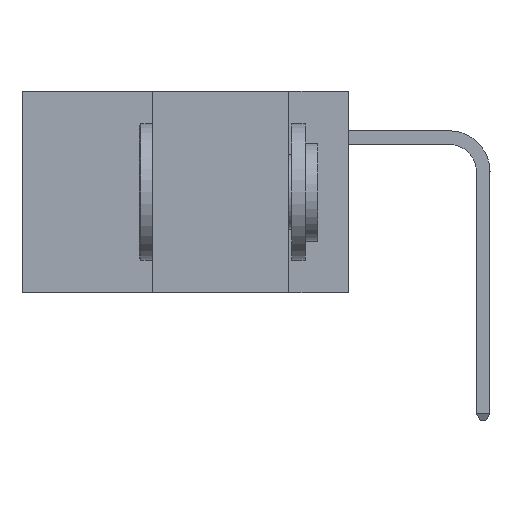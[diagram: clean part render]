
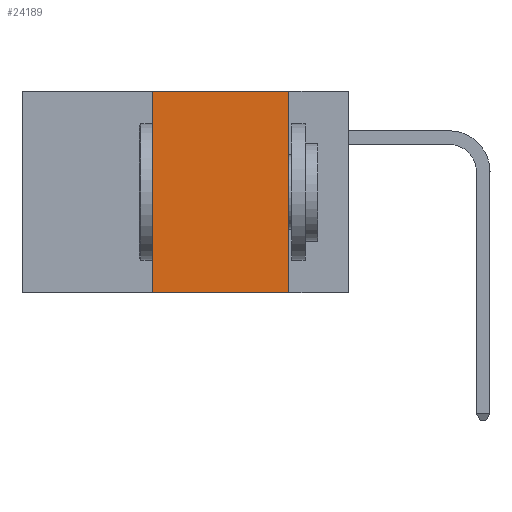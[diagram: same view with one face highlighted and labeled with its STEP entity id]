
A CAD part, left-side view. The second image highlights one B-rep face of the part: STEP entity #24189.
In plain terms, the highlighted planar face has unit normal (-1, 0, 0).
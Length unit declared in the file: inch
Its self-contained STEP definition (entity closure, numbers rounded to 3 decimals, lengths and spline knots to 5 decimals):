
#2197 = DIRECTION ( 'NONE',  ( 1., 0., 0. ) ) ;
#2327 = AXIS2_PLACEMENT_3D ( 'NONE', #24510, #2197, #20277 ) ;
#2576 = CARTESIAN_POINT ( 'NONE',  ( 0., 0.36, -0.37 ) ) ;
#3992 = PLANE ( 'NONE',  #2327 ) ;
#4759 = EDGE_CURVE ( 'NONE', #23033, #25270, #12099, .T. ) ;
#6342 = VERTEX_POINT ( 'NONE', #2576 ) ;
#7003 = DIRECTION ( 'NONE',  ( 0., 0., -1. ) ) ;
#7301 = CARTESIAN_POINT ( 'NONE',  ( 0., 0.36, 0. ) ) ;
#8258 = LINE ( 'NONE', #9106, #24716 ) ;
#8738 = ORIENTED_EDGE ( 'NONE', *, *, #17795, .F. ) ;
#9106 = CARTESIAN_POINT ( 'NONE',  ( 0., 0.36, 0. ) ) ;
#10291 = CARTESIAN_POINT ( 'NONE',  ( 0., 0.11, 0. ) ) ;
#10486 = ORIENTED_EDGE ( 'NONE', *, *, #16826, .F. ) ;
#11129 = VECTOR ( 'NONE', #7003, 39.37008 ) ;
#11482 = LINE ( 'NONE', #12072, #14945 ) ;
#11607 = CARTESIAN_POINT ( 'NONE',  ( 0., 0.6, -0.37 ) ) ;
#12072 = CARTESIAN_POINT ( 'NONE',  ( 0., 0.6, 0. ) ) ;
#12099 = LINE ( 'NONE', #10291, #11129 ) ;
#13743 = ORIENTED_EDGE ( 'NONE', *, *, #24019, .T. ) ;
#14022 = DIRECTION ( 'NONE',  ( 0., -1., 0. ) ) ;
#14323 = FACE_OUTER_BOUND ( 'NONE', #18024, .T. ) ;
#14945 = VECTOR ( 'NONE', #14022, 39.37008 ) ;
#15354 = ORIENTED_EDGE ( 'NONE', *, *, #4759, .F. ) ;
#15773 = CARTESIAN_POINT ( 'NONE',  ( 0., 0.11, -0.37 ) ) ;
#16826 = EDGE_CURVE ( 'NONE', #20624, #23033, #11482, .T. ) ;
#17795 = EDGE_CURVE ( 'NONE', #6342, #20624, #8258, .T. ) ;
#17899 = DIRECTION ( 'NONE',  ( 0., -1., 0. ) ) ;
#18024 = EDGE_LOOP ( 'NONE', ( #15354, #10486, #8738, #13743 ) ) ;
#19957 = CARTESIAN_POINT ( 'NONE',  ( 0., 0.11, 0. ) ) ;
#20277 = DIRECTION ( 'NONE',  ( 0., 0., -1. ) ) ;
#20624 = VERTEX_POINT ( 'NONE', #7301 ) ;
#21620 = VECTOR ( 'NONE', #17899, 39.37008 ) ;
#23033 = VERTEX_POINT ( 'NONE', #19957 ) ;
#24019 = EDGE_CURVE ( 'NONE', #6342, #25270, #25092, .T. ) ;
#24189 = ADVANCED_FACE ( 'NONE', ( #14323 ), #3992, .F. ) ;
#24510 = CARTESIAN_POINT ( 'NONE',  ( 0., 0.6, 0. ) ) ;
#24716 = VECTOR ( 'NONE', #25116, 39.37008 ) ;
#25092 = LINE ( 'NONE', #11607, #21620 ) ;
#25116 = DIRECTION ( 'NONE',  ( 0., 0., 1. ) ) ;
#25270 = VERTEX_POINT ( 'NONE', #15773 ) ;
